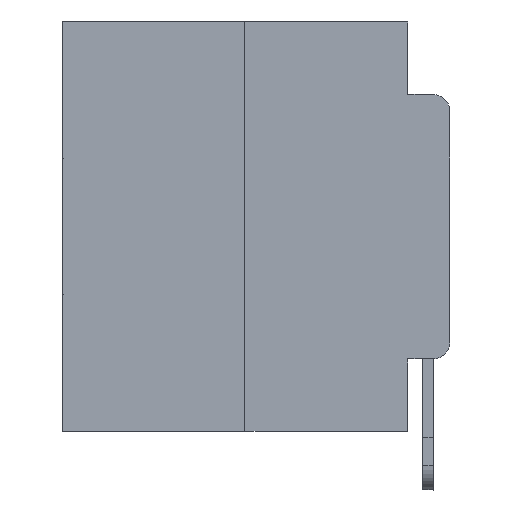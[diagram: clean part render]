
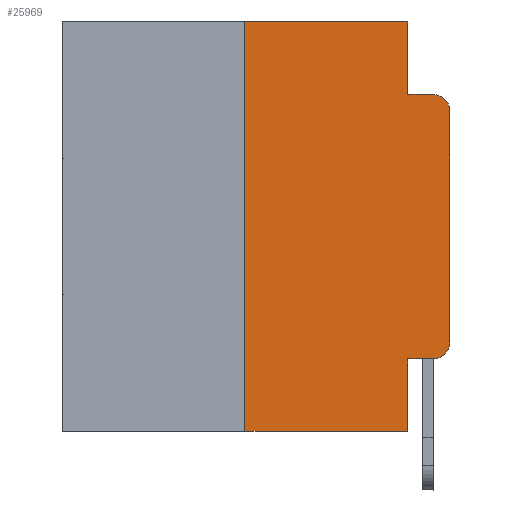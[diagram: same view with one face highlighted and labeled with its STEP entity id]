
A CAD part, left-side view. The second image highlights one B-rep face of the part: STEP entity #25969.
In plain terms, the highlighted planar face has unit normal (-1, 0, 0).
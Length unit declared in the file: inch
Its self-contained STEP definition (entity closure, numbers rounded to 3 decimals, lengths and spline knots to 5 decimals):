
#39 = VECTOR ( 'NONE', #11294, 39.37008 ) ;
#71 = DIRECTION ( 'NONE',  ( 0., 0., -1. ) ) ;
#154 = ORIENTED_EDGE ( 'NONE', *, *, #28313, .F. ) ;
#169 = DIRECTION ( 'NONE',  ( 1., 0., 0. ) ) ;
#424 = CIRCLE ( 'NONE', #12006, 0.02 ) ;
#734 = VECTOR ( 'NONE', #25867, 39.37008 ) ;
#1749 = CARTESIAN_POINT ( 'NONE',  ( 0., 0.02, -0.0885 ) ) ;
#2237 = DIRECTION ( 'NONE',  ( -1., 0., 0. ) ) ;
#2715 = DIRECTION ( 'NONE',  ( 0., 0., 1. ) ) ;
#2730 = ORIENTED_EDGE ( 'NONE', *, *, #10804, .F. ) ;
#2862 = EDGE_CURVE ( 'NONE', #11975, #6512, #20874, .T. ) ;
#2869 = VERTEX_POINT ( 'NONE', #3507 ) ;
#2999 = LINE ( 'NONE', #25005, #39 ) ;
#3507 = CARTESIAN_POINT ( 'NONE',  ( 0., 0., -0.1085 ) ) ;
#3982 = VECTOR ( 'NONE', #16590, 39.37008 ) ;
#4025 = VERTEX_POINT ( 'NONE', #4637 ) ;
#4185 = EDGE_CURVE ( 'NONE', #4025, #12836, #424, .T. ) ;
#4208 = VERTEX_POINT ( 'NONE', #10853 ) ;
#4319 = EDGE_CURVE ( 'NONE', #18159, #4208, #2999, .T. ) ;
#4592 = VECTOR ( 'NONE', #25776, 39.37008 ) ;
#4637 = CARTESIAN_POINT ( 'NONE',  ( 0., 0.02, -0.4115 ) ) ;
#4856 = CARTESIAN_POINT ( 'NONE',  ( 0., 0.051, -0.0885 ) ) ;
#5531 = EDGE_CURVE ( 'NONE', #12836, #2869, #15768, .T. ) ;
#5582 = CARTESIAN_POINT ( 'NONE',  ( 0., 0.051, 0. ) ) ;
#5778 = ORIENTED_EDGE ( 'NONE', *, *, #21641, .T. ) ;
#5947 = LINE ( 'NONE', #25627, #26712 ) ;
#6512 = VERTEX_POINT ( 'NONE', #7133 ) ;
#6517 = LINE ( 'NONE', #11034, #26335 ) ;
#7095 = FACE_OUTER_BOUND ( 'NONE', #26826, .T. ) ;
#7133 = CARTESIAN_POINT ( 'NONE',  ( 0., 0.051, 0. ) ) ;
#7138 = VECTOR ( 'NONE', #24554, 39.37008 ) ;
#7824 = CARTESIAN_POINT ( 'NONE',  ( 0., 0.25, -0.5 ) ) ;
#9225 = LINE ( 'NONE', #20060, #7138 ) ;
#9894 = CARTESIAN_POINT ( 'NONE',  ( 0., 0.473, 0. ) ) ;
#10804 = EDGE_CURVE ( 'NONE', #26379, #15894, #5947, .T. ) ;
#10853 = CARTESIAN_POINT ( 'NONE',  ( 0., 0.051, -0.5 ) ) ;
#11001 = DIRECTION ( 'NONE',  ( 0., 0., -1. ) ) ;
#11034 = CARTESIAN_POINT ( 'NONE',  ( 0., 0.051, 0. ) ) ;
#11294 = DIRECTION ( 'NONE',  ( 0., -1., 0. ) ) ;
#11358 = CIRCLE ( 'NONE', #21974, 0.02 ) ;
#11606 = ORIENTED_EDGE ( 'NONE', *, *, #4319, .T. ) ;
#11903 = ORIENTED_EDGE ( 'NONE', *, *, #22755, .F. ) ;
#11975 = VERTEX_POINT ( 'NONE', #20442 ) ;
#12006 = AXIS2_PLACEMENT_3D ( 'NONE', #21838, #17490, #11001 ) ;
#12275 = LINE ( 'NONE', #5582, #3982 ) ;
#12312 = LINE ( 'NONE', #27739, #734 ) ;
#12836 = VERTEX_POINT ( 'NONE', #19022 ) ;
#12980 = CARTESIAN_POINT ( 'NONE',  ( 0., 0.02, -0.1085 ) ) ;
#13246 = ORIENTED_EDGE ( 'NONE', *, *, #18192, .T. ) ;
#13550 = ORIENTED_EDGE ( 'NONE', *, *, #22294, .F. ) ;
#13764 = CARTESIAN_POINT ( 'NONE',  ( 0., 0., 0. ) ) ;
#14195 = ORIENTED_EDGE ( 'NONE', *, *, #4185, .T. ) ;
#15063 = ORIENTED_EDGE ( 'NONE', *, *, #5531, .T. ) ;
#15642 = CARTESIAN_POINT ( 'NONE',  ( 0., 0.051, -0.4115 ) ) ;
#15768 = LINE ( 'NONE', #13764, #18953 ) ;
#15894 = VERTEX_POINT ( 'NONE', #1749 ) ;
#16590 = DIRECTION ( 'NONE',  ( 0., 0., -1. ) ) ;
#16622 = PLANE ( 'NONE',  #17920 ) ;
#16682 = DIRECTION ( 'NONE',  ( 0., -1., 0. ) ) ;
#17343 = ORIENTED_EDGE ( 'NONE', *, *, #2862, .F. ) ;
#17490 = DIRECTION ( 'NONE',  ( -1., 0., 0. ) ) ;
#17920 = AXIS2_PLACEMENT_3D ( 'NONE', #22577, #169, #24897 ) ;
#18159 = VERTEX_POINT ( 'NONE', #7824 ) ;
#18192 = EDGE_CURVE ( 'NONE', #23868, #4025, #9225, .T. ) ;
#18953 = VECTOR ( 'NONE', #2715, 39.37008 ) ;
#19022 = CARTESIAN_POINT ( 'NONE',  ( 0., 0., -0.3915 ) ) ;
#20060 = CARTESIAN_POINT ( 'NONE',  ( 0., 0.051, -0.4115 ) ) ;
#20442 = CARTESIAN_POINT ( 'NONE',  ( 0., 0.25, 0. ) ) ;
#20874 = LINE ( 'NONE', #9894, #4592 ) ;
#21641 = EDGE_CURVE ( 'NONE', #2869, #15894, #11358, .T. ) ;
#21838 = CARTESIAN_POINT ( 'NONE',  ( 0., 0.02, -0.3915 ) ) ;
#21974 = AXIS2_PLACEMENT_3D ( 'NONE', #12980, #2237, #71 ) ;
#22008 = DIRECTION ( 'NONE',  ( 0., 0., -1. ) ) ;
#22294 = EDGE_CURVE ( 'NONE', #18159, #11975, #12312, .T. ) ;
#22577 = CARTESIAN_POINT ( 'NONE',  ( 0., 0.473, 0. ) ) ;
#22755 = EDGE_CURVE ( 'NONE', #23868, #4208, #12275, .T. ) ;
#23868 = VERTEX_POINT ( 'NONE', #15642 ) ;
#24554 = DIRECTION ( 'NONE',  ( 0., -1., 0. ) ) ;
#24897 = DIRECTION ( 'NONE',  ( 0., 0., -1. ) ) ;
#25005 = CARTESIAN_POINT ( 'NONE',  ( 0., 0.473, -0.5 ) ) ;
#25627 = CARTESIAN_POINT ( 'NONE',  ( 0., 0.051, -0.0885 ) ) ;
#25776 = DIRECTION ( 'NONE',  ( 0., -1., 0. ) ) ;
#25867 = DIRECTION ( 'NONE',  ( 0., 0., 1. ) ) ;
#25969 = ADVANCED_FACE ( 'NONE', ( #7095 ), #16622, .F. ) ;
#26335 = VECTOR ( 'NONE', #22008, 39.37008 ) ;
#26379 = VERTEX_POINT ( 'NONE', #4856 ) ;
#26712 = VECTOR ( 'NONE', #16682, 39.37008 ) ;
#26826 = EDGE_LOOP ( 'NONE', ( #15063, #5778, #2730, #154, #17343, #13550, #11606, #11903, #13246, #14195 ) ) ;
#27739 = CARTESIAN_POINT ( 'NONE',  ( 0., 0.25, 0. ) ) ;
#28313 = EDGE_CURVE ( 'NONE', #6512, #26379, #6517, .T. ) ;
